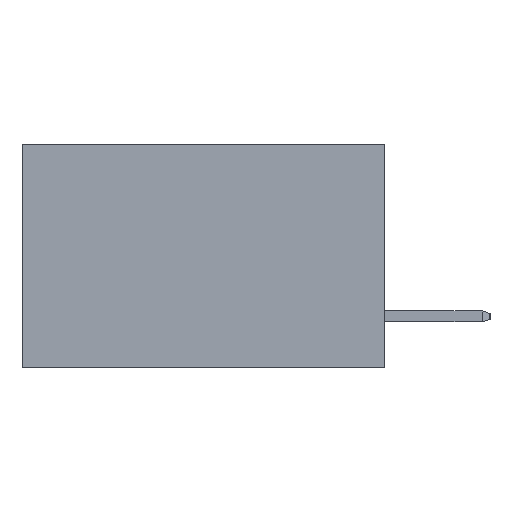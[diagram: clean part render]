
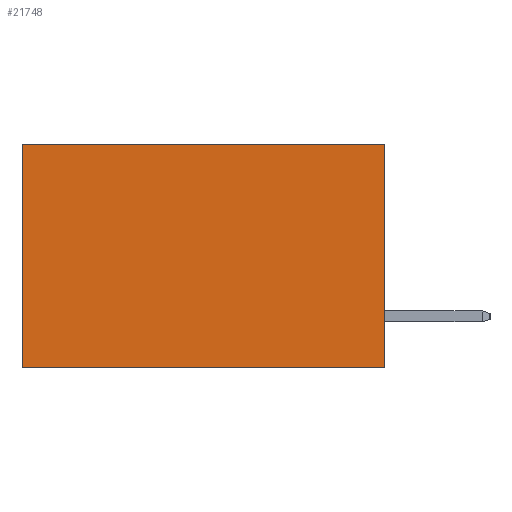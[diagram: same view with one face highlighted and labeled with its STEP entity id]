
A CAD part, left-side view. The second image highlights one B-rep face of the part: STEP entity #21748.
In plain terms, the highlighted planar face has unit normal (-1, 0, 0).
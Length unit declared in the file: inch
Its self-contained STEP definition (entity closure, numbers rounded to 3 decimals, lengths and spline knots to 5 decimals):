
#2012 = FACE_OUTER_BOUND ( 'NONE', #7165, .T. ) ;
#2904 = LINE ( 'NONE', #10079, #17608 ) ;
#3593 = PLANE ( 'NONE',  #11673 ) ;
#3677 = DIRECTION ( 'NONE',  ( 1., 0., 0. ) ) ;
#4841 = DIRECTION ( 'NONE',  ( 0., 0., -1. ) ) ;
#4945 = CARTESIAN_POINT ( 'NONE',  ( 0.2615, 0.6, -0.37 ) ) ;
#6427 = ORIENTED_EDGE ( 'NONE', *, *, #8401, .T. ) ;
#7082 = DIRECTION ( 'NONE',  ( 0., 1., 0. ) ) ;
#7165 = EDGE_LOOP ( 'NONE', ( #7810, #19141, #11637, #6427 ) ) ;
#7166 = VECTOR ( 'NONE', #4841, 39.37008 ) ;
#7198 = CARTESIAN_POINT ( 'NONE',  ( 0.2615, 0., 0. ) ) ;
#7810 = ORIENTED_EDGE ( 'NONE', *, *, #8364, .T. ) ;
#8364 = EDGE_CURVE ( 'NONE', #10618, #21382, #12258, .T. ) ;
#8401 = EDGE_CURVE ( 'NONE', #16340, #10618, #20491, .T. ) ;
#8534 = EDGE_CURVE ( 'NONE', #16261, #21382, #2904, .T. ) ;
#9532 = CARTESIAN_POINT ( 'NONE',  ( 0.2615, 0., -0.37 ) ) ;
#9607 = DIRECTION ( 'NONE',  ( 0., 1., 0. ) ) ;
#10079 = CARTESIAN_POINT ( 'NONE',  ( 0.2615, 0., -0.37 ) ) ;
#10618 = VERTEX_POINT ( 'NONE', #19913 ) ;
#11637 = ORIENTED_EDGE ( 'NONE', *, *, #13539, .F. ) ;
#11673 = AXIS2_PLACEMENT_3D ( 'NONE', #9532, #3677, #22657 ) ;
#12258 = LINE ( 'NONE', #4945, #7166 ) ;
#13539 = EDGE_CURVE ( 'NONE', #16340, #16261, #21692, .T. ) ;
#14668 = CARTESIAN_POINT ( 'NONE',  ( 0.2615, 0., 0. ) ) ;
#16177 = CARTESIAN_POINT ( 'NONE',  ( 0.2615, 0.6, -0.37 ) ) ;
#16261 = VERTEX_POINT ( 'NONE', #16378 ) ;
#16340 = VERTEX_POINT ( 'NONE', #14668 ) ;
#16378 = CARTESIAN_POINT ( 'NONE',  ( 0.2615, 0., -0.37 ) ) ;
#17608 = VECTOR ( 'NONE', #9607, 39.37008 ) ;
#19141 = ORIENTED_EDGE ( 'NONE', *, *, #8534, .F. ) ;
#19913 = CARTESIAN_POINT ( 'NONE',  ( 0.2615, 0.6, 0. ) ) ;
#20491 = LINE ( 'NONE', #7198, #21062 ) ;
#21062 = VECTOR ( 'NONE', #7082, 39.37008 ) ;
#21091 = DIRECTION ( 'NONE',  ( 0., 0., -1. ) ) ;
#21109 = CARTESIAN_POINT ( 'NONE',  ( 0.2615, 0., -0.37 ) ) ;
#21382 = VERTEX_POINT ( 'NONE', #16177 ) ;
#21692 = LINE ( 'NONE', #21109, #22275 ) ;
#21748 = ADVANCED_FACE ( 'NONE', ( #2012 ), #3593, .F. ) ;
#22275 = VECTOR ( 'NONE', #21091, 39.37008 ) ;
#22657 = DIRECTION ( 'NONE',  ( 0., 0., -1. ) ) ;
